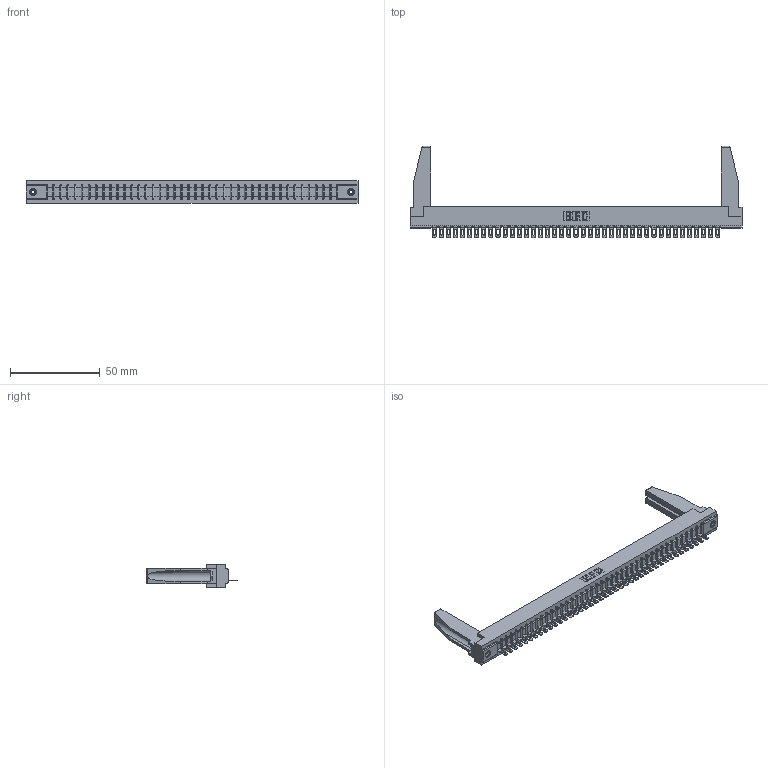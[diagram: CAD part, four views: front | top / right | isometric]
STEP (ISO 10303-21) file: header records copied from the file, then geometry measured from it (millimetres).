
FILE_DESCRIPTION (( 'STEP AP203' ), '1' );
FILE_NAME ('357-041-501-178.STEP', '2019-09-17T09:32:38', ( '' ), ( '' ), 'SwSTEP 2.0', 'SolidWorks 2016', '' );
FILE_SCHEMA (( 'CONFIG_CONTROL_DESIGN' ));
Length unit declared in the file: inch
Products named in the file (5): 307 Part_.156 Dia Mounting Holes; 345-250-001_345-250-001-102; 307-290-002_501; 357-041-501-178; 307-220-078
Assembly tree (46 placements, depth 2):
  357-041-501-178
    307 Part_.156 Dia Mounting Holes
    307-290-002_501  x41
    307-220-078  x2
    345-250-001_345-250-001-102  x2
Bounding box: 185.47 x 51.13 x 12.7 mm (x, y, z)
Volume: 23869.3 mm3; surface area: 29071.5 mm2
Topology: 46 solids, 46 shells, 3406 faces, 10411 edges, 6818 vertices
Faces by surface type: plane 1958, cylinder 1348, sphere 84, cone 12, torus 4
Entity records: 38505 total; most frequent: CARTESIAN_POINT 6494, ORIENTED_EDGE 6440, DIRECTION 6270, EDGE_CURVE 3220, VECTOR 2466, LINE 2466, VERTEX_POINT 2084, AXIS2_PLACEMENT_3D 1902
